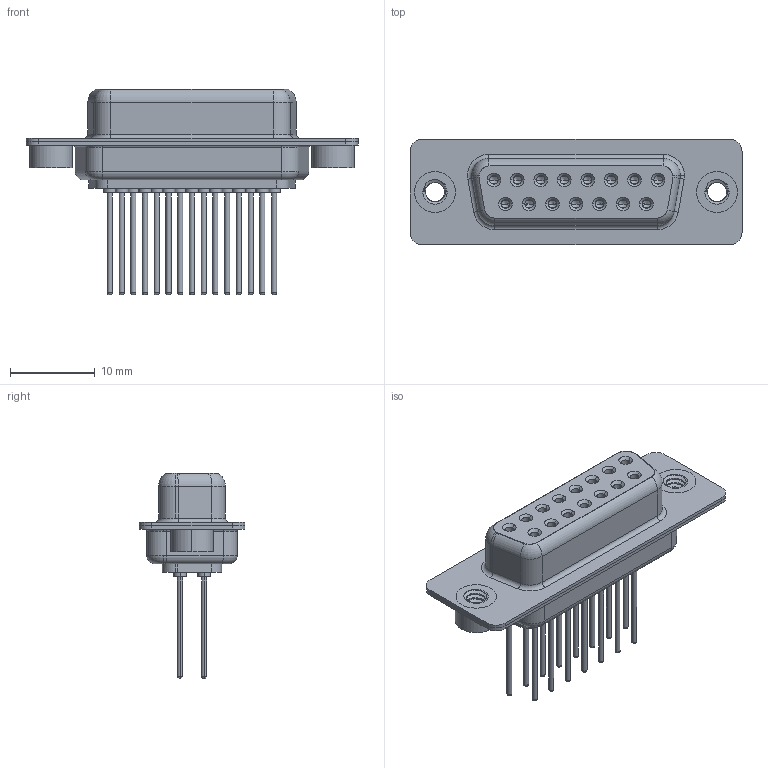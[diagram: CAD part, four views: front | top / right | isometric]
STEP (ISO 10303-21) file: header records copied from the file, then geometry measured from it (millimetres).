
FILE_DESCRIPTION (( 'STEP AP203' ), '1' );
FILE_NAME ('628-M15-223-BT2.STEP', '2020-07-16T21:46:20', ( '' ), ( '' ), 'SwSTEP 2.0', 'SolidWorks 2020', '' );
FILE_SCHEMA (( 'CONFIG_CONTROL_DESIGN' ));
Length unit declared in the file: millimetre
Products named in the file (7): 628M Shell Rear_15 Contacts; 628M Housing_15 Contacts; 628M Shell Front_15 Contacts; 628M 4-40 Threaded Rivet; 628M Contact Row 1_23; 628-M15-223-BT2; 628M Contact Row 2_23
Assembly tree (20 placements, depth 2):
  628-M15-223-BT2
    628M Housing_15 Contacts
    628M Shell Front_15 Contacts
    628M Shell Rear_15 Contacts
    628M Contact Row 1_23  x8
    628M Contact Row 2_23  x7
    628M 4-40 Threaded Rivet  x2
Bounding box: 39.2 x 12.5 x 24.27 mm (x, y, z)
Volume: 2500.9 mm3; surface area: 6392.8 mm2
Topology: 20 solids, 20 shells, 1104 faces, 2577 edges, 1584 vertices
Faces by surface type: cylinder 422, plane 292, torus 273, cone 111, bspline 6
Entity records: 17856 total; most frequent: CARTESIAN_POINT 4265, DIRECTION 2883, ORIENTED_EDGE 2434, EDGE_CURVE 1217, AXIS2_PLACEMENT_3D 1216, VERTEX_POINT 764, CIRCLE 671, EDGE_LOOP 629
